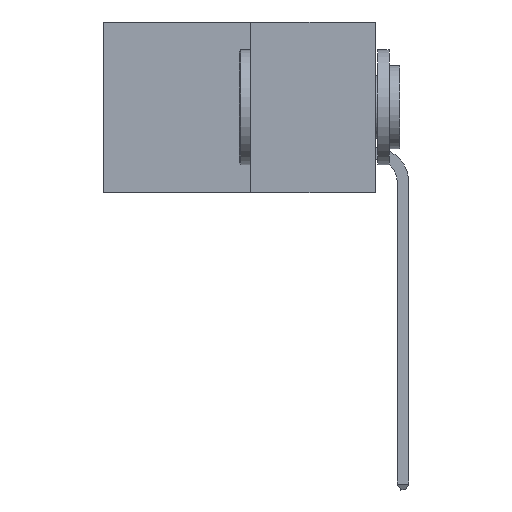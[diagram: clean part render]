
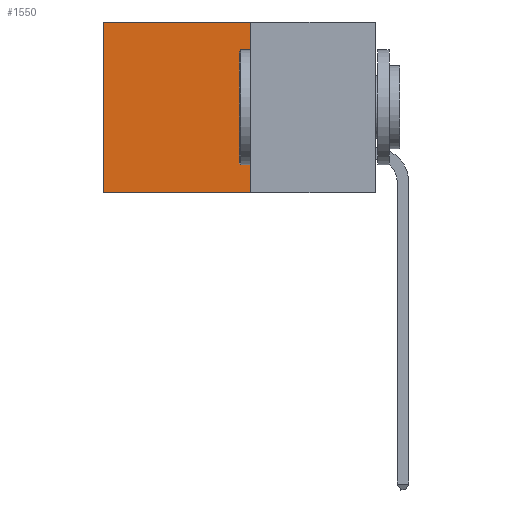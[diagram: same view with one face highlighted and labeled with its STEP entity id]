
A CAD part, left-side view. The second image highlights one B-rep face of the part: STEP entity #1550.
In plain terms, the highlighted planar face has unit normal (-1, 0, 0).
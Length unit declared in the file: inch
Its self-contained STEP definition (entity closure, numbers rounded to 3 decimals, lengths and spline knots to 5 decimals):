
#431 = CARTESIAN_POINT ( 'NONE',  ( 0.277, 0.27, -0.37 ) ) ;
#506 = AXIS2_PLACEMENT_3D ( 'NONE', #5057, #2530, #1293 ) ;
#518 = VECTOR ( 'NONE', #1319, 39.37008 ) ;
#1057 = ORIENTED_EDGE ( 'NONE', *, *, #1535, .F. ) ;
#1293 = DIRECTION ( 'NONE',  ( 0., 0., -1. ) ) ;
#1319 = DIRECTION ( 'NONE',  ( 0., 1., 0. ) ) ;
#1324 = EDGE_CURVE ( 'NONE', #3576, #4914, #2570, .T. ) ;
#1535 = EDGE_CURVE ( 'NONE', #4914, #6218, #6667, .T. ) ;
#1550 = ADVANCED_FACE ( 'NONE', ( #2993 ), #4100, .F. ) ;
#2318 = LINE ( 'NONE', #3119, #5815 ) ;
#2527 = CARTESIAN_POINT ( 'NONE',  ( 0.277, 0.59, -0.37 ) ) ;
#2530 = DIRECTION ( 'NONE',  ( 1., 0., 0. ) ) ;
#2560 = DIRECTION ( 'NONE',  ( 0., 1., 0. ) ) ;
#2570 = LINE ( 'NONE', #4921, #3773 ) ;
#2590 = LINE ( 'NONE', #8708, #518 ) ;
#2591 = ORIENTED_EDGE ( 'NONE', *, *, #1324, .F. ) ;
#2604 = ORIENTED_EDGE ( 'NONE', *, *, #7076, .T. ) ;
#2993 = FACE_OUTER_BOUND ( 'NONE', #4489, .T. ) ;
#3064 = DIRECTION ( 'NONE',  ( 0., 0., -1. ) ) ;
#3119 = CARTESIAN_POINT ( 'NONE',  ( 0.277, 0.59, -0.37 ) ) ;
#3462 = CARTESIAN_POINT ( 'NONE',  ( 0.277, 0.27, -0.37 ) ) ;
#3576 = VERTEX_POINT ( 'NONE', #8642 ) ;
#3773 = VECTOR ( 'NONE', #4728, 39.37008 ) ;
#4100 = PLANE ( 'NONE',  #506 ) ;
#4114 = EDGE_CURVE ( 'NONE', #7494, #6218, #2318, .T. ) ;
#4489 = EDGE_LOOP ( 'NONE', ( #7665, #1057, #2591, #2604 ) ) ;
#4728 = DIRECTION ( 'NONE',  ( 0., 0., -1. ) ) ;
#4890 = VECTOR ( 'NONE', #2560, 39.37008 ) ;
#4914 = VERTEX_POINT ( 'NONE', #431 ) ;
#4921 = CARTESIAN_POINT ( 'NONE',  ( 0.277, 0.27, -0.37 ) ) ;
#5057 = CARTESIAN_POINT ( 'NONE',  ( 0.277, 0.27, -0.37 ) ) ;
#5815 = VECTOR ( 'NONE', #3064, 39.37008 ) ;
#6218 = VERTEX_POINT ( 'NONE', #2527 ) ;
#6667 = LINE ( 'NONE', #3462, #4890 ) ;
#6674 = CARTESIAN_POINT ( 'NONE',  ( 0.277, 0.59, 0. ) ) ;
#7076 = EDGE_CURVE ( 'NONE', #3576, #7494, #2590, .T. ) ;
#7494 = VERTEX_POINT ( 'NONE', #6674 ) ;
#7665 = ORIENTED_EDGE ( 'NONE', *, *, #4114, .T. ) ;
#8642 = CARTESIAN_POINT ( 'NONE',  ( 0.277, 0.27, 0. ) ) ;
#8708 = CARTESIAN_POINT ( 'NONE',  ( 0.277, 0.27, 0. ) ) ;
